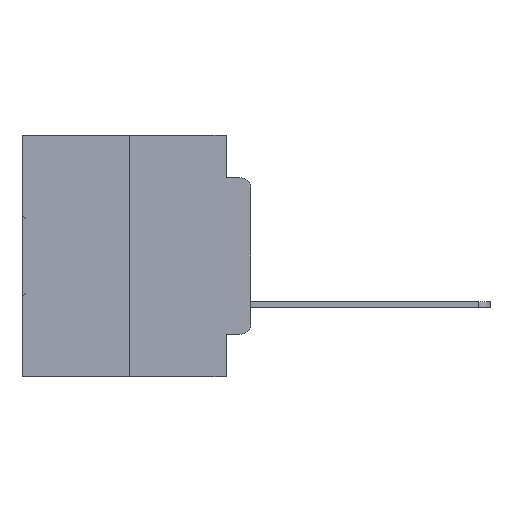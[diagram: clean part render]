
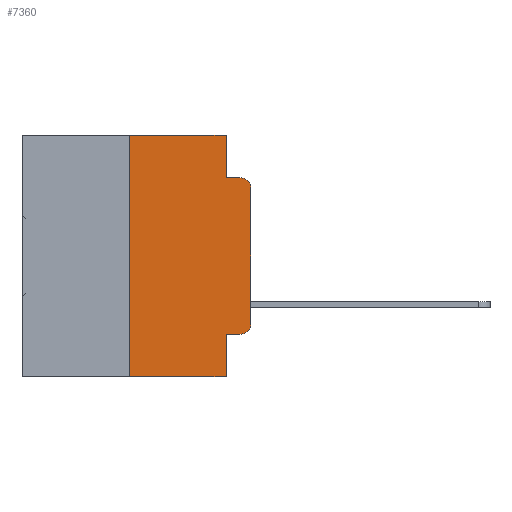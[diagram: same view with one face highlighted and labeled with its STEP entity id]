
A CAD part, left-side view. The second image highlights one B-rep face of the part: STEP entity #7360.
In plain terms, the highlighted planar face has unit normal (-1, 0, 0).
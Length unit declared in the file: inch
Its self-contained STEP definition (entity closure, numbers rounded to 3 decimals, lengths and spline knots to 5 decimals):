
#1705 = ORIENTED_EDGE ( 'NONE', *, *, #1790, .T. ) ;
#1790 = EDGE_CURVE ( 'NONE', #24558, #21643, #21962, .T. ) ;
#1950 = ORIENTED_EDGE ( 'NONE', *, *, #32978, .T. ) ;
#2152 = CARTESIAN_POINT ( 'NONE',  ( 0., 0.051, -0.4115 ) ) ;
#2607 = EDGE_CURVE ( 'NONE', #17650, #5352, #6392, .T. ) ;
#2865 = ORIENTED_EDGE ( 'NONE', *, *, #2607, .F. ) ;
#2894 = CARTESIAN_POINT ( 'NONE',  ( 0., 0.25, -0.5 ) ) ;
#3005 = VERTEX_POINT ( 'NONE', #4529 ) ;
#3189 = CARTESIAN_POINT ( 'NONE',  ( 0., 0.25, 0. ) ) ;
#3793 = CARTESIAN_POINT ( 'NONE',  ( 0., 0.473, -0.5 ) ) ;
#3924 = LINE ( 'NONE', #23067, #10827 ) ;
#4028 = ORIENTED_EDGE ( 'NONE', *, *, #21269, .F. ) ;
#4189 = ORIENTED_EDGE ( 'NONE', *, *, #34412, .T. ) ;
#4384 = CARTESIAN_POINT ( 'NONE',  ( 0., 0.473, 0. ) ) ;
#4529 = CARTESIAN_POINT ( 'NONE',  ( 0., 0.02, -0.0885 ) ) ;
#4637 = DIRECTION ( 'NONE',  ( 0., 0., 1. ) ) ;
#4857 = ORIENTED_EDGE ( 'NONE', *, *, #17799, .F. ) ;
#5352 = VERTEX_POINT ( 'NONE', #11569 ) ;
#5459 = ORIENTED_EDGE ( 'NONE', *, *, #14159, .T. ) ;
#6392 = LINE ( 'NONE', #15549, #26939 ) ;
#6648 = ORIENTED_EDGE ( 'NONE', *, *, #28094, .F. ) ;
#6688 = ORIENTED_EDGE ( 'NONE', *, *, #8586, .T. ) ;
#7360 = ADVANCED_FACE ( 'NONE', ( #13025 ), #7439, .F. ) ;
#7439 = PLANE ( 'NONE',  #18439 ) ;
#8358 = AXIS2_PLACEMENT_3D ( 'NONE', #29816, #14412, #32279 ) ;
#8586 = EDGE_CURVE ( 'NONE', #30609, #24558, #20450, .T. ) ;
#9696 = DIRECTION ( 'NONE',  ( 0., -1., 0. ) ) ;
#10167 = ORIENTED_EDGE ( 'NONE', *, *, #26435, .F. ) ;
#10234 = CARTESIAN_POINT ( 'NONE',  ( 0., 0., 0. ) ) ;
#10325 = DIRECTION ( 'NONE',  ( 0., 0., -1. ) ) ;
#10827 = VECTOR ( 'NONE', #9696, 39.37008 ) ;
#10846 = DIRECTION ( 'NONE',  ( 0., 0., -1. ) ) ;
#10949 = LINE ( 'NONE', #34010, #24314 ) ;
#11569 = CARTESIAN_POINT ( 'NONE',  ( 0., 0.051, 0. ) ) ;
#12119 = LINE ( 'NONE', #14450, #12987 ) ;
#12987 = VECTOR ( 'NONE', #17178, 39.37008 ) ;
#13025 = FACE_OUTER_BOUND ( 'NONE', #14077, .T. ) ;
#13203 = DIRECTION ( 'NONE',  ( -1., 0., 0. ) ) ;
#13851 = VECTOR ( 'NONE', #19852, 39.37008 ) ;
#14077 = EDGE_LOOP ( 'NONE', ( #1705, #1950, #6648, #10167, #2865, #4028, #4189, #4857, #5459, #6688 ) ) ;
#14159 = EDGE_CURVE ( 'NONE', #18213, #30609, #3924, .T. ) ;
#14412 = DIRECTION ( 'NONE',  ( -1., 0., 0. ) ) ;
#14450 = CARTESIAN_POINT ( 'NONE',  ( 0., 0.051, 0. ) ) ;
#14662 = CARTESIAN_POINT ( 'NONE',  ( 0., 0.051, -0.5 ) ) ;
#14818 = VERTEX_POINT ( 'NONE', #26483 ) ;
#14902 = CARTESIAN_POINT ( 'NONE',  ( 0., 0., -0.3915 ) ) ;
#15337 = AXIS2_PLACEMENT_3D ( 'NONE', #28772, #13203, #31244 ) ;
#15549 = CARTESIAN_POINT ( 'NONE',  ( 0., 0.473, 0. ) ) ;
#17178 = DIRECTION ( 'NONE',  ( 0., 0., -1. ) ) ;
#17650 = VERTEX_POINT ( 'NONE', #34013 ) ;
#17772 = CIRCLE ( 'NONE', #15337, 0.02 ) ;
#17799 = EDGE_CURVE ( 'NONE', #18213, #24537, #12119, .T. ) ;
#18213 = VERTEX_POINT ( 'NONE', #2152 ) ;
#18439 = AXIS2_PLACEMENT_3D ( 'NONE', #4384, #26180, #10325 ) ;
#18841 = CARTESIAN_POINT ( 'NONE',  ( 0., 0., -0.1085 ) ) ;
#19852 = DIRECTION ( 'NONE',  ( 0., -1., 0. ) ) ;
#20450 = CIRCLE ( 'NONE', #8358, 0.02 ) ;
#21269 = EDGE_CURVE ( 'NONE', #25918, #17650, #22873, .T. ) ;
#21532 = DIRECTION ( 'NONE',  ( 0., -1., 0. ) ) ;
#21643 = VERTEX_POINT ( 'NONE', #18841 ) ;
#21962 = LINE ( 'NONE', #10234, #23112 ) ;
#22873 = LINE ( 'NONE', #3189, #29484 ) ;
#23067 = CARTESIAN_POINT ( 'NONE',  ( 0., 0.051, -0.4115 ) ) ;
#23112 = VECTOR ( 'NONE', #4637, 39.37008 ) ;
#24314 = VECTOR ( 'NONE', #10846, 39.37008 ) ;
#24537 = VERTEX_POINT ( 'NONE', #14662 ) ;
#24558 = VERTEX_POINT ( 'NONE', #14902 ) ;
#25395 = LINE ( 'NONE', #32454, #13851 ) ;
#25918 = VERTEX_POINT ( 'NONE', #2894 ) ;
#26180 = DIRECTION ( 'NONE',  ( 1., 0., 0. ) ) ;
#26435 = EDGE_CURVE ( 'NONE', #5352, #14818, #10949, .T. ) ;
#26483 = CARTESIAN_POINT ( 'NONE',  ( 0., 0.051, -0.0885 ) ) ;
#26939 = VECTOR ( 'NONE', #21532, 39.37008 ) ;
#27167 = CARTESIAN_POINT ( 'NONE',  ( 0., 0.02, -0.4115 ) ) ;
#28094 = EDGE_CURVE ( 'NONE', #14818, #3005, #25395, .T. ) ;
#28772 = CARTESIAN_POINT ( 'NONE',  ( 0., 0.02, -0.1085 ) ) ;
#29484 = VECTOR ( 'NONE', #30017, 39.37008 ) ;
#29816 = CARTESIAN_POINT ( 'NONE',  ( 0., 0.02, -0.3915 ) ) ;
#30017 = DIRECTION ( 'NONE',  ( 0., 0., 1. ) ) ;
#30609 = VERTEX_POINT ( 'NONE', #27167 ) ;
#31244 = DIRECTION ( 'NONE',  ( 0., 0., -1. ) ) ;
#32279 = DIRECTION ( 'NONE',  ( 0., 0., -1. ) ) ;
#32454 = CARTESIAN_POINT ( 'NONE',  ( 0., 0.051, -0.0885 ) ) ;
#32961 = DIRECTION ( 'NONE',  ( 0., -1., 0. ) ) ;
#32978 = EDGE_CURVE ( 'NONE', #21643, #3005, #17772, .T. ) ;
#33774 = VECTOR ( 'NONE', #32961, 39.37008 ) ;
#34010 = CARTESIAN_POINT ( 'NONE',  ( 0., 0.051, 0. ) ) ;
#34013 = CARTESIAN_POINT ( 'NONE',  ( 0., 0.25, 0. ) ) ;
#34412 = EDGE_CURVE ( 'NONE', #25918, #24537, #34557, .T. ) ;
#34557 = LINE ( 'NONE', #3793, #33774 ) ;
